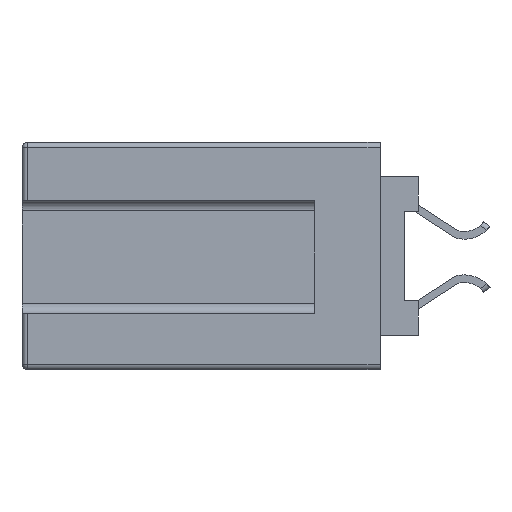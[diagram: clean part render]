
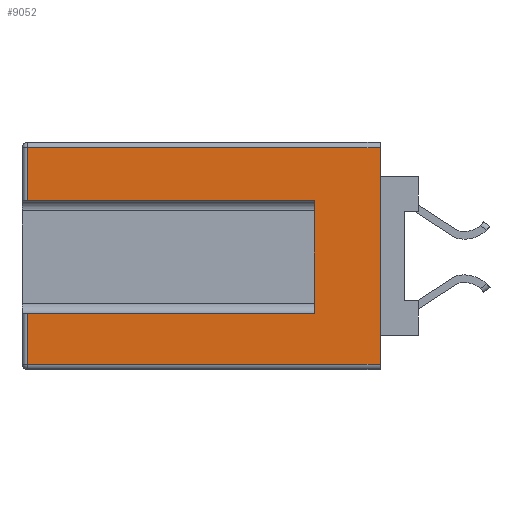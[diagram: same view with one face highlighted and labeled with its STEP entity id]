
A CAD part, left-side view. The second image highlights one B-rep face of the part: STEP entity #9052.
In plain terms, the highlighted planar face has unit normal (-1, 0, 0).
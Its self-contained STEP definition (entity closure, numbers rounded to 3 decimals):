
#809 = DIRECTION ( 'NONE',  ( 0., 0., -1. ) ) ;
#1002 = ORIENTED_EDGE ( 'NONE', *, *, #21312, .T. ) ;
#1054 = LINE ( 'NONE', #4121, #37169 ) ;
#1427 = EDGE_CURVE ( 'NONE', #26307, #13539, #24957, .T. ) ;
#1672 = CARTESIAN_POINT ( 'NONE',  ( 0., 1.5, -8.68 ) ) ;
#1745 = EDGE_CURVE ( 'NONE', #15618, #26307, #34916, .T. ) ;
#2281 = DIRECTION ( 'NONE',  ( 0., -1., 0. ) ) ;
#4121 = CARTESIAN_POINT ( 'NONE',  ( 0., 4.07, -2.28 ) ) ;
#4284 = VERTEX_POINT ( 'NONE', #5701 ) ;
#4350 = CARTESIAN_POINT ( 'NONE',  ( 0., 15.3, -0.2 ) ) ;
#4684 = CARTESIAN_POINT ( 'NONE',  ( 0., 15.3, -6.68 ) ) ;
#5701 = CARTESIAN_POINT ( 'NONE',  ( 0., 4.07, -2.28 ) ) ;
#6286 = LINE ( 'NONE', #7060, #9879 ) ;
#6378 = CARTESIAN_POINT ( 'NONE',  ( 0., 1.5, 0. ) ) ;
#6745 = EDGE_LOOP ( 'NONE', ( #14455, #1002, #31289, #12780, #16506, #8910, #18562, #19105 ) ) ;
#7060 = CARTESIAN_POINT ( 'NONE',  ( 0., 15.5, -0.2 ) ) ;
#7564 = DIRECTION ( 'NONE',  ( 0., 0., -1. ) ) ;
#8197 = VERTEX_POINT ( 'NONE', #10455 ) ;
#8200 = PLANE ( 'NONE',  #30630 ) ;
#8355 = CARTESIAN_POINT ( 'NONE',  ( 0., 4.07, -6.68 ) ) ;
#8910 = ORIENTED_EDGE ( 'NONE', *, *, #17410, .T. ) ;
#9052 = ADVANCED_FACE ( 'NONE', ( #34969 ), #8200, .F. ) ;
#9879 = VECTOR ( 'NONE', #9947, 1000. ) ;
#9947 = DIRECTION ( 'NONE',  ( 0., 1., 0. ) ) ;
#10455 = CARTESIAN_POINT ( 'NONE',  ( 0., 1.5, -0.2 ) ) ;
#11086 = EDGE_CURVE ( 'NONE', #4284, #15618, #1054, .T. ) ;
#12780 = ORIENTED_EDGE ( 'NONE', *, *, #16605, .T. ) ;
#13324 = LINE ( 'NONE', #36821, #37128 ) ;
#13539 = VERTEX_POINT ( 'NONE', #36362 ) ;
#14455 = ORIENTED_EDGE ( 'NONE', *, *, #1427, .T. ) ;
#15020 = VECTOR ( 'NONE', #2281, 1000. ) ;
#15333 = VERTEX_POINT ( 'NONE', #4350 ) ;
#15618 = VERTEX_POINT ( 'NONE', #32608 ) ;
#16484 = VERTEX_POINT ( 'NONE', #33239 ) ;
#16506 = ORIENTED_EDGE ( 'NONE', *, *, #31723, .T. ) ;
#16605 = EDGE_CURVE ( 'NONE', #8197, #15333, #6286, .T. ) ;
#17410 = EDGE_CURVE ( 'NONE', #16484, #4284, #32297, .T. ) ;
#18562 = ORIENTED_EDGE ( 'NONE', *, *, #11086, .T. ) ;
#19105 = ORIENTED_EDGE ( 'NONE', *, *, #1745, .T. ) ;
#19900 = VECTOR ( 'NONE', #35905, 1000. ) ;
#19972 = CARTESIAN_POINT ( 'NONE',  ( 0., 15.5, 0. ) ) ;
#21312 = EDGE_CURVE ( 'NONE', #13539, #34622, #13324, .T. ) ;
#23501 = VECTOR ( 'NONE', #27643, 1000. ) ;
#24957 = LINE ( 'NONE', #33598, #19900 ) ;
#26307 = VERTEX_POINT ( 'NONE', #4684 ) ;
#27464 = LINE ( 'NONE', #36481, #23501 ) ;
#27643 = DIRECTION ( 'NONE',  ( 0., 0., -1. ) ) ;
#28945 = DIRECTION ( 'NONE',  ( 0., 1., 0. ) ) ;
#29225 = CARTESIAN_POINT ( 'NONE',  ( 0., 4.07, -2.28 ) ) ;
#29893 = EDGE_CURVE ( 'NONE', #8197, #34622, #30066, .T. ) ;
#30066 = LINE ( 'NONE', #6378, #36712 ) ;
#30630 = AXIS2_PLACEMENT_3D ( 'NONE', #19972, #31710, #37661 ) ;
#31046 = DIRECTION ( 'NONE',  ( 0., -1., 0. ) ) ;
#31289 = ORIENTED_EDGE ( 'NONE', *, *, #29893, .F. ) ;
#31710 = DIRECTION ( 'NONE',  ( 1., 0., 0. ) ) ;
#31723 = EDGE_CURVE ( 'NONE', #15333, #16484, #27464, .T. ) ;
#32297 = LINE ( 'NONE', #29225, #15020 ) ;
#32608 = CARTESIAN_POINT ( 'NONE',  ( 0., 4.07, -6.68 ) ) ;
#33239 = CARTESIAN_POINT ( 'NONE',  ( 0., 15.3, -2.28 ) ) ;
#33259 = VECTOR ( 'NONE', #28945, 1000. ) ;
#33598 = CARTESIAN_POINT ( 'NONE',  ( 0., 15.3, 0. ) ) ;
#34622 = VERTEX_POINT ( 'NONE', #1672 ) ;
#34916 = LINE ( 'NONE', #8355, #33259 ) ;
#34969 = FACE_OUTER_BOUND ( 'NONE', #6745, .T. ) ;
#35905 = DIRECTION ( 'NONE',  ( 0., 0., -1. ) ) ;
#36362 = CARTESIAN_POINT ( 'NONE',  ( 0., 15.3, -8.68 ) ) ;
#36481 = CARTESIAN_POINT ( 'NONE',  ( 0., 15.3, 0. ) ) ;
#36712 = VECTOR ( 'NONE', #809, 1000. ) ;
#36821 = CARTESIAN_POINT ( 'NONE',  ( 0., 15.5, -8.68 ) ) ;
#37128 = VECTOR ( 'NONE', #31046, 1000. ) ;
#37169 = VECTOR ( 'NONE', #7564, 1000. ) ;
#37661 = DIRECTION ( 'NONE',  ( 0., 0., -1. ) ) ;
